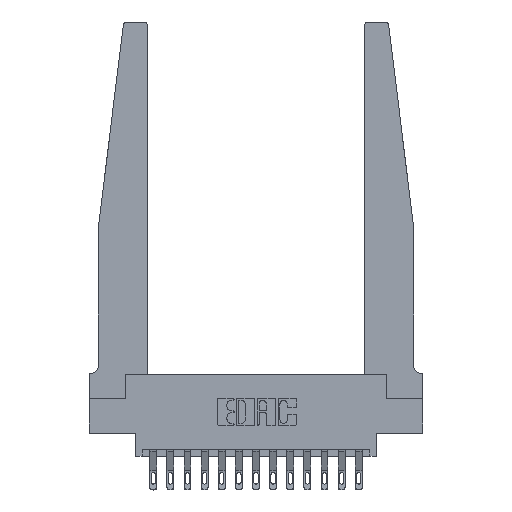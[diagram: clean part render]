
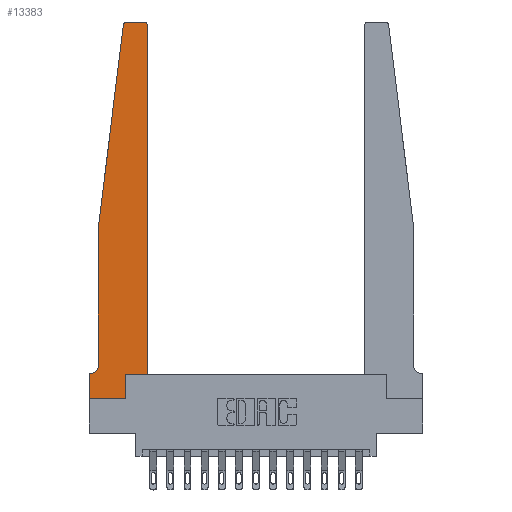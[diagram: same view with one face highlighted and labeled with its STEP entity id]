
A CAD part, top view. The second image highlights one B-rep face of the part: STEP entity #13383.
In plain terms, the highlighted planar face has unit normal (0, 0, 1).
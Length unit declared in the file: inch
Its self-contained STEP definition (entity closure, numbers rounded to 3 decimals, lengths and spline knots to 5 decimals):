
#89 = DIRECTION ( 'NONE',  ( 1., 0., 0. ) ) ;
#158 = CARTESIAN_POINT ( 'NONE',  ( 0.015, 0.2375, 0.37 ) ) ;
#212 = CARTESIAN_POINT ( 'NONE',  ( 0.425, 2.72, 0.37 ) ) ;
#492 = DIRECTION ( 'NONE',  ( -1., 0., 0. ) ) ;
#595 = ORIENTED_EDGE ( 'NONE', *, *, #6500, .T. ) ;
#690 = CARTESIAN_POINT ( 'NONE',  ( 0., 0.1875, 0.37 ) ) ;
#718 = VERTEX_POINT ( 'NONE', #9771 ) ;
#849 = EDGE_CURVE ( 'NONE', #15338, #12744, #8028, .T. ) ;
#1287 = ORIENTED_EDGE ( 'NONE', *, *, #1304, .T. ) ;
#1304 = EDGE_CURVE ( 'NONE', #9588, #6477, #13524, .T. ) ;
#1542 = DIRECTION ( 'NONE',  ( -1., 0., 0. ) ) ;
#1568 = CARTESIAN_POINT ( 'NONE',  ( 0.2605, 0.18, 0.37 ) ) ;
#1753 = CARTESIAN_POINT ( 'NONE',  ( 0.065, 1.25, 0.37 ) ) ;
#1807 = DIRECTION ( 'NONE',  ( 1., 0., 0. ) ) ;
#1876 = CARTESIAN_POINT ( 'NONE',  ( 0.425, 0.18, 0.37 ) ) ;
#2101 = DIRECTION ( 'NONE',  ( 1., 0., 0. ) ) ;
#2114 = EDGE_CURVE ( 'NONE', #7091, #4199, #15677, .T. ) ;
#2160 = VECTOR ( 'NONE', #12507, 39.37008 ) ;
#2183 = CARTESIAN_POINT ( 'NONE',  ( 0., 0.1875, 0.37 ) ) ;
#2209 = LINE ( 'NONE', #13465, #9040 ) ;
#2324 = ORIENTED_EDGE ( 'NONE', *, *, #2114, .T. ) ;
#2418 = CIRCLE ( 'NONE', #10603, 0.03 ) ;
#2534 = AXIS2_PLACEMENT_3D ( 'NONE', #690, #10268, #2101 ) ;
#2855 = LINE ( 'NONE', #9072, #16840 ) ;
#3110 = VECTOR ( 'NONE', #14950, 39.37008 ) ;
#3236 = EDGE_CURVE ( 'NONE', #5003, #9588, #17084, .T. ) ;
#3274 = DIRECTION ( 'NONE',  ( 1., 0., 0. ) ) ;
#3613 = ORIENTED_EDGE ( 'NONE', *, *, #5002, .T. ) ;
#4199 = VERTEX_POINT ( 'NONE', #2183 ) ;
#4537 = VERTEX_POINT ( 'NONE', #212 ) ;
#4647 = DIRECTION ( 'NONE',  ( 0., 0., 1. ) ) ;
#4754 = LINE ( 'NONE', #13394, #7970 ) ;
#4906 = AXIS2_PLACEMENT_3D ( 'NONE', #158, #9755, #1542 ) ;
#4959 = DIRECTION ( 'NONE',  ( 0., -1., 0. ) ) ;
#5002 = EDGE_CURVE ( 'NONE', #718, #4537, #2209, .T. ) ;
#5003 = VERTEX_POINT ( 'NONE', #5326 ) ;
#5326 = CARTESIAN_POINT ( 'NONE',  ( 0.395, 2.75, 0.37 ) ) ;
#5357 = EDGE_CURVE ( 'NONE', #5532, #16247, #4754, .T. ) ;
#5532 = VERTEX_POINT ( 'NONE', #12375 ) ;
#5951 = EDGE_LOOP ( 'NONE', ( #12107, #1287, #6045, #13228, #9280, #2324, #13681, #6136, #595, #12050, #3613, #16217 ) ) ;
#6045 = ORIENTED_EDGE ( 'NONE', *, *, #12540, .T. ) ;
#6136 = ORIENTED_EDGE ( 'NONE', *, *, #849, .T. ) ;
#6477 = VERTEX_POINT ( 'NONE', #8347 ) ;
#6500 = EDGE_CURVE ( 'NONE', #12744, #16960, #13020, .T. ) ;
#6627 = CIRCLE ( 'NONE', #4906, 0.05 ) ;
#6699 = DIRECTION ( 'NONE',  ( 0., 1., 0. ) ) ;
#6963 = CARTESIAN_POINT ( 'NONE',  ( 0.015, 0.1875, 0.37 ) ) ;
#7091 = VERTEX_POINT ( 'NONE', #6963 ) ;
#7325 = CARTESIAN_POINT ( 'NONE',  ( 0.065, 0.2375, 0.37 ) ) ;
#7766 = CARTESIAN_POINT ( 'NONE',  ( 0., 0., 0.37 ) ) ;
#7970 = VECTOR ( 'NONE', #7992, 39.37008 ) ;
#7992 = DIRECTION ( 'NONE',  ( 0., -1., 0. ) ) ;
#8028 = LINE ( 'NONE', #11348, #11197 ) ;
#8313 = DIRECTION ( 'NONE',  ( 0., 0., 1. ) ) ;
#8347 = CARTESIAN_POINT ( 'NONE',  ( 0.24675, 2.72367, 0.37 ) ) ;
#8909 = PLANE ( 'NONE',  #2534 ) ;
#9040 = VECTOR ( 'NONE', #6699, 39.37008 ) ;
#9072 = CARTESIAN_POINT ( 'NONE',  ( 0., 0., 0.37 ) ) ;
#9280 = ORIENTED_EDGE ( 'NONE', *, *, #11271, .T. ) ;
#9588 = VERTEX_POINT ( 'NONE', #10486 ) ;
#9755 = DIRECTION ( 'NONE',  ( 0., 0., -1. ) ) ;
#9771 = CARTESIAN_POINT ( 'NONE',  ( 0.425, 0.18, 0.37 ) ) ;
#9955 = DIRECTION ( 'NONE',  ( -0.122, -0.992, 0. ) ) ;
#10097 = EDGE_CURVE ( 'NONE', #16960, #718, #17235, .T. ) ;
#10268 = DIRECTION ( 'NONE',  ( 0., 0., 1. ) ) ;
#10486 = CARTESIAN_POINT ( 'NONE',  ( 0.27653, 2.75, 0.37 ) ) ;
#10603 = AXIS2_PLACEMENT_3D ( 'NONE', #12804, #4647, #14176 ) ;
#11197 = VECTOR ( 'NONE', #1807, 39.37008 ) ;
#11248 = LINE ( 'NONE', #1753, #14871 ) ;
#11271 = EDGE_CURVE ( 'NONE', #16247, #7091, #6627, .T. ) ;
#11348 = CARTESIAN_POINT ( 'NONE',  ( 0., 0., 0.37 ) ) ;
#12050 = ORIENTED_EDGE ( 'NONE', *, *, #10097, .T. ) ;
#12085 = VECTOR ( 'NONE', #492, 39.37008 ) ;
#12107 = ORIENTED_EDGE ( 'NONE', *, *, #3236, .T. ) ;
#12375 = CARTESIAN_POINT ( 'NONE',  ( 0.065, 1.25, 0.37 ) ) ;
#12507 = DIRECTION ( 'NONE',  ( 0., 1., 0. ) ) ;
#12540 = EDGE_CURVE ( 'NONE', #6477, #5532, #11248, .T. ) ;
#12744 = VERTEX_POINT ( 'NONE', #14394 ) ;
#12804 = CARTESIAN_POINT ( 'NONE',  ( 0.395, 2.72, 0.37 ) ) ;
#12927 = FACE_OUTER_BOUND ( 'NONE', #5951, .T. ) ;
#13020 = LINE ( 'NONE', #1568, #2160 ) ;
#13208 = CARTESIAN_POINT ( 'NONE',  ( 0.2605, 0.18, 0.37 ) ) ;
#13228 = ORIENTED_EDGE ( 'NONE', *, *, #5357, .T. ) ;
#13383 = ADVANCED_FACE ( 'NONE', ( #12927 ), #8909, .T. ) ;
#13394 = CARTESIAN_POINT ( 'NONE',  ( 0.065, 1.25, 0.37 ) ) ;
#13465 = CARTESIAN_POINT ( 'NONE',  ( 0.425, 0.18, 0.37 ) ) ;
#13524 = CIRCLE ( 'NONE', #13922, 0.03 ) ;
#13681 = ORIENTED_EDGE ( 'NONE', *, *, #15303, .T. ) ;
#13922 = AXIS2_PLACEMENT_3D ( 'NONE', #16405, #8313, #89 ) ;
#14176 = DIRECTION ( 'NONE',  ( 1., 0., 0. ) ) ;
#14394 = CARTESIAN_POINT ( 'NONE',  ( 0.2605, 0., 0.37 ) ) ;
#14871 = VECTOR ( 'NONE', #9955, 39.37008 ) ;
#14950 = DIRECTION ( 'NONE',  ( -1., 0., 0. ) ) ;
#15303 = EDGE_CURVE ( 'NONE', #4199, #15338, #2855, .T. ) ;
#15338 = VERTEX_POINT ( 'NONE', #7766 ) ;
#15677 = LINE ( 'NONE', #16781, #12085 ) ;
#16217 = ORIENTED_EDGE ( 'NONE', *, *, #17494, .T. ) ;
#16247 = VERTEX_POINT ( 'NONE', #7325 ) ;
#16405 = CARTESIAN_POINT ( 'NONE',  ( 0.27653, 2.72, 0.37 ) ) ;
#16781 = CARTESIAN_POINT ( 'NONE',  ( 0.065, 0.1875, 0.37 ) ) ;
#16807 = VECTOR ( 'NONE', #3274, 39.37008 ) ;
#16840 = VECTOR ( 'NONE', #4959, 39.37008 ) ;
#16960 = VERTEX_POINT ( 'NONE', #13208 ) ;
#17084 = LINE ( 'NONE', #17571, #3110 ) ;
#17235 = LINE ( 'NONE', #1876, #16807 ) ;
#17494 = EDGE_CURVE ( 'NONE', #4537, #5003, #2418, .T. ) ;
#17571 = CARTESIAN_POINT ( 'NONE',  ( 0.25, 2.75, 0.37 ) ) ;
